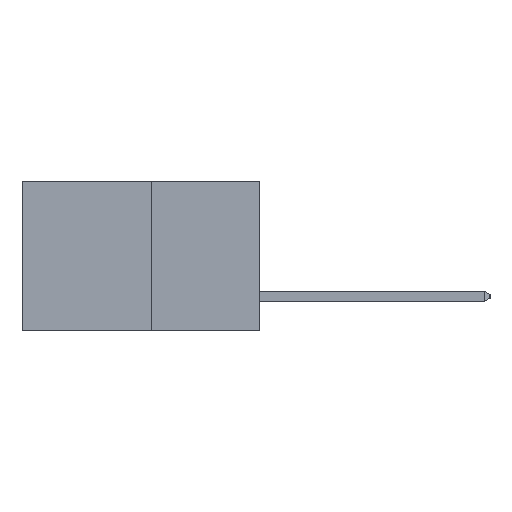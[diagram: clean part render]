
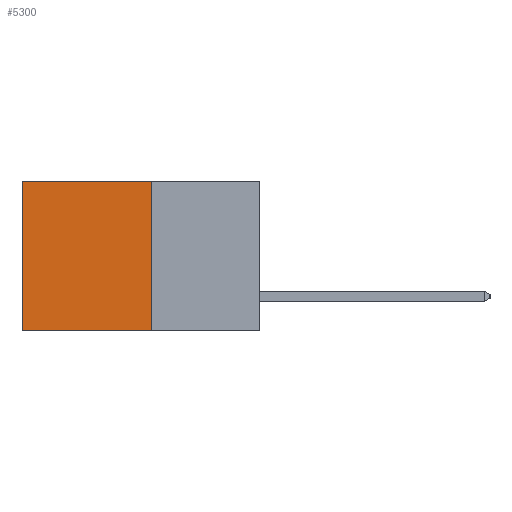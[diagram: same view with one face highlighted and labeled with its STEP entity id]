
A CAD part, left-side view. The second image highlights one B-rep face of the part: STEP entity #5300.
In plain terms, the highlighted planar face has unit normal (-1, 0, 0).
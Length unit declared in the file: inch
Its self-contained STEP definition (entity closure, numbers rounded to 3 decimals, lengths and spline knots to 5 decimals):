
#88 = CARTESIAN_POINT ( 'NONE',  ( 0.277, 0.27, -0.37 ) ) ;
#204 = VECTOR ( 'NONE', #7157, 39.37008 ) ;
#304 = ORIENTED_EDGE ( 'NONE', *, *, #3510, .T. ) ;
#308 = DIRECTION ( 'NONE',  ( 1., 0., 0. ) ) ;
#524 = CARTESIAN_POINT ( 'NONE',  ( 0.277, 0.59, 0. ) ) ;
#721 = ORIENTED_EDGE ( 'NONE', *, *, #3105, .F. ) ;
#1065 = CARTESIAN_POINT ( 'NONE',  ( 0.277, 0.27, 0. ) ) ;
#1171 = EDGE_LOOP ( 'NONE', ( #304, #7388, #721, #1713 ) ) ;
#1197 = LINE ( 'NONE', #8195, #6422 ) ;
#1571 = CARTESIAN_POINT ( 'NONE',  ( 0.277, 0.59, -0.37 ) ) ;
#1612 = VERTEX_POINT ( 'NONE', #8244 ) ;
#1689 = DIRECTION ( 'NONE',  ( 0., 1., 0. ) ) ;
#1713 = ORIENTED_EDGE ( 'NONE', *, *, #4865, .T. ) ;
#1850 = DIRECTION ( 'NONE',  ( 0., 0., -1. ) ) ;
#2234 = PLANE ( 'NONE',  #7279 ) ;
#2625 = VERTEX_POINT ( 'NONE', #1065 ) ;
#2963 = LINE ( 'NONE', #5623, #204 ) ;
#3105 = EDGE_CURVE ( 'NONE', #2625, #1612, #8294, .T. ) ;
#3510 = EDGE_CURVE ( 'NONE', #4640, #6676, #5416, .T. ) ;
#4479 = CARTESIAN_POINT ( 'NONE',  ( 0.277, 0.59, -0.37 ) ) ;
#4640 = VERTEX_POINT ( 'NONE', #524 ) ;
#4865 = EDGE_CURVE ( 'NONE', #2625, #4640, #2963, .T. ) ;
#4991 = EDGE_CURVE ( 'NONE', #1612, #6676, #1197, .T. ) ;
#5077 = CARTESIAN_POINT ( 'NONE',  ( 0.277, 0.27, -0.37 ) ) ;
#5216 = DIRECTION ( 'NONE',  ( 0., 0., -1. ) ) ;
#5300 = ADVANCED_FACE ( 'NONE', ( #5698 ), #2234, .F. ) ;
#5416 = LINE ( 'NONE', #4479, #8468 ) ;
#5623 = CARTESIAN_POINT ( 'NONE',  ( 0.277, 0.27, 0. ) ) ;
#5698 = FACE_OUTER_BOUND ( 'NONE', #1171, .T. ) ;
#6422 = VECTOR ( 'NONE', #1689, 39.37008 ) ;
#6552 = VECTOR ( 'NONE', #8355, 39.37008 ) ;
#6676 = VERTEX_POINT ( 'NONE', #1571 ) ;
#7157 = DIRECTION ( 'NONE',  ( 0., 1., 0. ) ) ;
#7279 = AXIS2_PLACEMENT_3D ( 'NONE', #88, #308, #1850 ) ;
#7388 = ORIENTED_EDGE ( 'NONE', *, *, #4991, .F. ) ;
#8195 = CARTESIAN_POINT ( 'NONE',  ( 0.277, 0.27, -0.37 ) ) ;
#8244 = CARTESIAN_POINT ( 'NONE',  ( 0.277, 0.27, -0.37 ) ) ;
#8294 = LINE ( 'NONE', #5077, #6552 ) ;
#8355 = DIRECTION ( 'NONE',  ( 0., 0., -1. ) ) ;
#8468 = VECTOR ( 'NONE', #5216, 39.37008 ) ;
